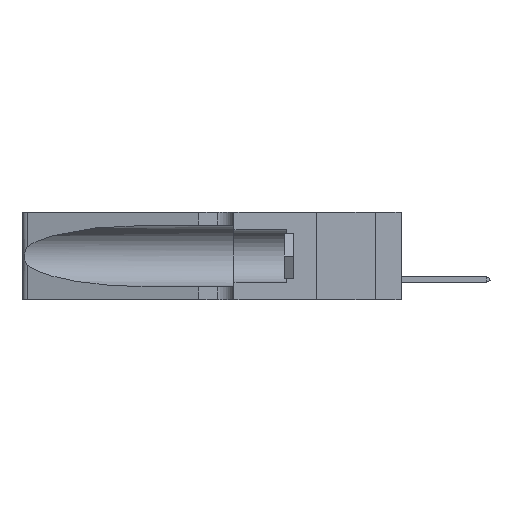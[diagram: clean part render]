
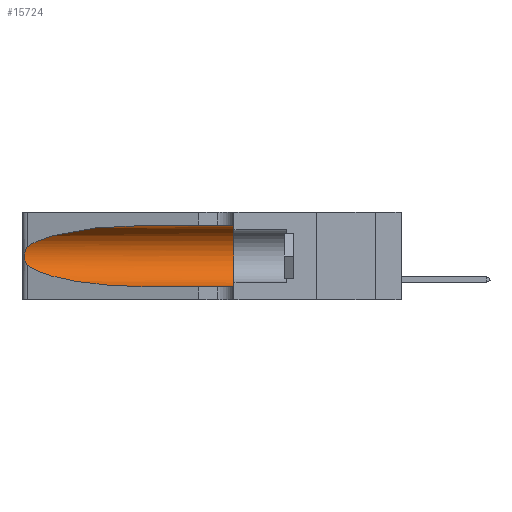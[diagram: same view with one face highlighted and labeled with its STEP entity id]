
A CAD part, left-side view. The second image highlights one B-rep face of the part: STEP entity #15724.
In plain terms, the highlighted cylindrical face has radius 3.308 mm (diameter 6.617 mm), a partial arc.
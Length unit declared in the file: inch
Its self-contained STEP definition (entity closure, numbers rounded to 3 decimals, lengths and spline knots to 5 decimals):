
#2154 = EDGE_CURVE ( 'NONE', #10304, #19830, #22762, .T. ) ;
#2270 = ORIENTED_EDGE ( 'NONE', *, *, #4538, .F. ) ;
#2485 = DIRECTION ( 'NONE',  ( 0., -1., 0. ) ) ;
#3140 = CARTESIAN_POINT ( 'NONE',  ( 0.25487, 1.22718, 0.22369 ) ) ;
#3263 = VERTEX_POINT ( 'NONE', #25432 ) ;
#3570 = CARTESIAN_POINT ( 'NONE',  ( 0.25639, 1.23186, 0.15144 ) ) ;
#3690 = CARTESIAN_POINT ( 'NONE',  ( 0.25856, 1.23593, 0.16098 ) ) ;
#4538 = EDGE_CURVE ( 'NONE', #3263, #10304, #24145, .T. ) ;
#4760 = VECTOR ( 'NONE', #26163, 39.37008 ) ;
#6277 = CARTESIAN_POINT ( 'NONE',  ( 0.25487, 1.22718, 0.22369 ) ) ;
#7700 = CARTESIAN_POINT ( 'NONE',  ( 0.1305, 0.35, 0.185 ) ) ;
#7851 = CARTESIAN_POINT ( 'NONE',  ( 0.26017, 1.23833, 0.17102 ) ) ;
#9513 = ORIENTED_EDGE ( 'NONE', *, *, #14116, .T. ) ;
#9658 = CARTESIAN_POINT ( 'NONE',  ( 0.25487, 1.22718, 0.14631 ) ) ;
#10156 = VERTEX_POINT ( 'NONE', #10346 ) ;
#10172 = FACE_OUTER_BOUND ( 'NONE', #20936, .T. ) ;
#10304 = VERTEX_POINT ( 'NONE', #27973 ) ;
#10346 = CARTESIAN_POINT ( 'NONE',  ( 0.1305, 0.72297, 0.05475 ) ) ;
#10836 = CARTESIAN_POINT ( 'NONE',  ( 0.25555, 1.22993, 0.14849 ) ) ;
#11041 = CARTESIAN_POINT ( 'NONE',  ( 0.25487, 1.22718, 0.14631 ) ) ;
#11943 = DIRECTION ( 'NONE',  ( 0., 1., 0. ) ) ;
#12032 =( BOUNDED_CURVE ( )  B_SPLINE_CURVE ( 3, ( #23719, #18124, #21440, #6277 ),
 .UNSPECIFIED., .F., .F. ) 
 B_SPLINE_CURVE_WITH_KNOTS ( ( 4, 4 ),
 ( 1.5708, 2.84003 ),
 .UNSPECIFIED. ) 
 CURVE ( )  GEOMETRIC_REPRESENTATION_ITEM ( )  RATIONAL_B_SPLINE_CURVE ( ( 1., 0.87, 0.87, 1. ) ) 
 REPRESENTATION_ITEM ( '' )  );
#12455 = DIRECTION ( 'NONE',  ( 0., 0., 1. ) ) ;
#12485 = CARTESIAN_POINT ( 'NONE',  ( 0.26075, 1.23896, 0.19203 ) ) ;
#12554 = ORIENTED_EDGE ( 'NONE', *, *, #2154, .F. ) ;
#14116 = EDGE_CURVE ( 'NONE', #28356, #10156, #17194, .T. ) ;
#14882 = VECTOR ( 'NONE', #25730, 39.37008 ) ;
#15724 = ADVANCED_FACE ( 'NONE', ( #10172 ), #17212, .F. ) ;
#16930 = CARTESIAN_POINT ( 'NONE',  ( 0.1305, 1.61858, 0.31525 ) ) ;
#17194 =( BOUNDED_CURVE ( )  B_SPLINE_CURVE ( 3, ( #9658, #20018, #24843, #29597 ),
 .UNSPECIFIED., .F., .T. ) 
 B_SPLINE_CURVE_WITH_KNOTS ( ( 4, 4 ),
 ( 3.44316, 4.71239 ),
 .UNSPECIFIED. ) 
 CURVE ( )  GEOMETRIC_REPRESENTATION_ITEM ( )  RATIONAL_B_SPLINE_CURVE ( ( 1., 0.87, 0.87, 1. ) ) 
 REPRESENTATION_ITEM ( '' )  );
#17212 = CYLINDRICAL_SURFACE ( 'NONE', #25847, 0.13025 ) ;
#17348 = CARTESIAN_POINT ( 'NONE',  ( 0.25487, 1.22718, 0.14631 ) ) ;
#17596 = B_SPLINE_CURVE_WITH_KNOTS ( 'NONE', 3,
 ( #19299, #19401, #24209, #27137, #29080, #21996, #12485, #19721, #7851, #3690, #27673, #3570, #10836, #11041 ),
 .UNSPECIFIED., .F., .F.,
 ( 4, 2, 2, 2, 2, 2, 4 ),
 ( 0., 0.00027, 0.00053, 0.00107, 0.0016, 0.00187, 0.00214 ),
 .UNSPECIFIED. ) ;
#18124 = CARTESIAN_POINT ( 'NONE',  ( 0.18966, 0.96281, 0.31525 ) ) ;
#19121 = CARTESIAN_POINT ( 'NONE',  ( 0.1305, 0.35, 0.05475 ) ) ;
#19213 = ORIENTED_EDGE ( 'NONE', *, *, #21502, .T. ) ;
#19299 = CARTESIAN_POINT ( 'NONE',  ( 0.25487, 1.22718, 0.22369 ) ) ;
#19401 = CARTESIAN_POINT ( 'NONE',  ( 0.25555, 1.22994, 0.2215 ) ) ;
#19721 = CARTESIAN_POINT ( 'NONE',  ( 0.26075, 1.23896, 0.178 ) ) ;
#19830 = VERTEX_POINT ( 'NONE', #19121 ) ;
#20018 = CARTESIAN_POINT ( 'NONE',  ( 0.2373, 1.15595, 0.08982 ) ) ;
#20074 = ORIENTED_EDGE ( 'NONE', *, *, #22082, .T. ) ;
#20259 = AXIS2_PLACEMENT_3D ( 'NONE', #7700, #11943, #12455 ) ;
#20936 = EDGE_LOOP ( 'NONE', ( #20074, #27785, #9513, #19213, #12554, #2270 ) ) ;
#21288 = LINE ( 'NONE', #30597, #14882 ) ;
#21440 = CARTESIAN_POINT ( 'NONE',  ( 0.2373, 1.15595, 0.28018 ) ) ;
#21502 = EDGE_CURVE ( 'NONE', #10156, #19830, #21288, .T. ) ;
#21996 = CARTESIAN_POINT ( 'NONE',  ( 0.26018, 1.23835, 0.19895 ) ) ;
#22082 = EDGE_CURVE ( 'NONE', #3263, #26719, #12032, .T. ) ;
#22762 = CIRCLE ( 'NONE', #20259, 0.13025 ) ;
#23719 = CARTESIAN_POINT ( 'NONE',  ( 0.1305, 0.72297, 0.31525 ) ) ;
#24145 = LINE ( 'NONE', #16930, #4760 ) ;
#24209 = CARTESIAN_POINT ( 'NONE',  ( 0.25639, 1.23184, 0.21858 ) ) ;
#24843 = CARTESIAN_POINT ( 'NONE',  ( 0.18966, 0.96281, 0.05475 ) ) ;
#25432 = CARTESIAN_POINT ( 'NONE',  ( 0.1305, 0.72297, 0.31525 ) ) ;
#25730 = DIRECTION ( 'NONE',  ( 0., -1., 0. ) ) ;
#25847 = AXIS2_PLACEMENT_3D ( 'NONE', #26658, #2485, #27744 ) ;
#26163 = DIRECTION ( 'NONE',  ( 0., -1., 0. ) ) ;
#26658 = CARTESIAN_POINT ( 'NONE',  ( 0.1305, 1.61858, 0.185 ) ) ;
#26719 = VERTEX_POINT ( 'NONE', #3140 ) ;
#27137 = CARTESIAN_POINT ( 'NONE',  ( 0.25787, 1.23484, 0.2124 ) ) ;
#27666 = EDGE_CURVE ( 'NONE', #26719, #28356, #17596, .T. ) ;
#27673 = CARTESIAN_POINT ( 'NONE',  ( 0.25789, 1.23486, 0.15765 ) ) ;
#27744 = DIRECTION ( 'NONE',  ( 0., 0., -1. ) ) ;
#27785 = ORIENTED_EDGE ( 'NONE', *, *, #27666, .T. ) ;
#27973 = CARTESIAN_POINT ( 'NONE',  ( 0.1305, 0.35, 0.31525 ) ) ;
#28356 = VERTEX_POINT ( 'NONE', #17348 ) ;
#29080 = CARTESIAN_POINT ( 'NONE',  ( 0.25854, 1.2359, 0.20912 ) ) ;
#29597 = CARTESIAN_POINT ( 'NONE',  ( 0.1305, 0.72297, 0.05475 ) ) ;
#30597 = CARTESIAN_POINT ( 'NONE',  ( 0.1305, 1.61858, 0.05475 ) ) ;
